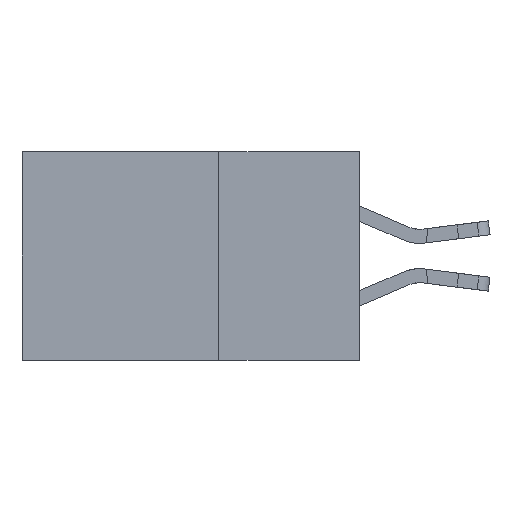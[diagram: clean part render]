
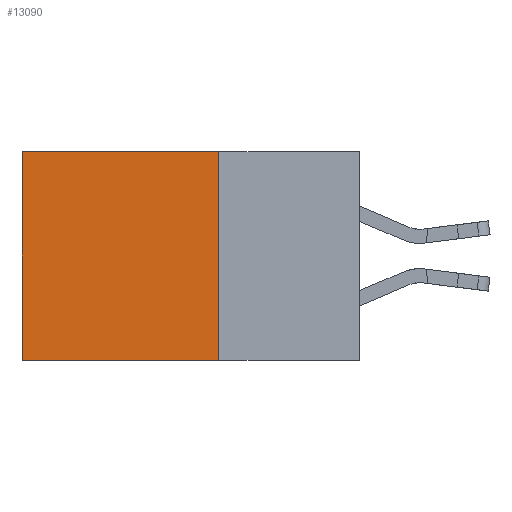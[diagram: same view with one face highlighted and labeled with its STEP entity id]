
A CAD part, left-side view. The second image highlights one B-rep face of the part: STEP entity #13090.
In plain terms, the highlighted planar face has unit normal (-1, 0, 0).
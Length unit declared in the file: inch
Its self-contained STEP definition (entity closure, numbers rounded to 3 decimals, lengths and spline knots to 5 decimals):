
#671 = CARTESIAN_POINT ( 'NONE',  ( 0.2875, 0.25, -0.37 ) ) ;
#3125 = DIRECTION ( 'NONE',  ( 0., 0., -1. ) ) ;
#3146 = VECTOR ( 'NONE', #27133, 39.37008 ) ;
#5110 = LINE ( 'NONE', #15081, #3146 ) ;
#6224 = LINE ( 'NONE', #28887, #25252 ) ;
#6437 = CARTESIAN_POINT ( 'NONE',  ( 0.2875, 0.25, 0. ) ) ;
#8980 = VERTEX_POINT ( 'NONE', #14138 ) ;
#8996 = PLANE ( 'NONE',  #17904 ) ;
#9022 = DIRECTION ( 'NONE',  ( 0., 1., 0. ) ) ;
#9914 = CARTESIAN_POINT ( 'NONE',  ( 0.2875, 0.6, 0. ) ) ;
#11239 = DIRECTION ( 'NONE',  ( 0., 0., -1. ) ) ;
#11529 = DIRECTION ( 'NONE',  ( 0., 0., -1. ) ) ;
#13090 = ADVANCED_FACE ( 'NONE', ( #13191 ), #8996, .F. ) ;
#13191 = FACE_OUTER_BOUND ( 'NONE', #18414, .T. ) ;
#14138 = CARTESIAN_POINT ( 'NONE',  ( 0.2875, 0.25, 0. ) ) ;
#14411 = ORIENTED_EDGE ( 'NONE', *, *, #16341, .T. ) ;
#15081 = CARTESIAN_POINT ( 'NONE',  ( 0.2875, 0.25, -0.37 ) ) ;
#16036 = CARTESIAN_POINT ( 'NONE',  ( 0.2875, 0.6, 0. ) ) ;
#16063 = VERTEX_POINT ( 'NONE', #16036 ) ;
#16341 = EDGE_CURVE ( 'NONE', #16063, #16381, #24700, .T. ) ;
#16381 = VERTEX_POINT ( 'NONE', #17940 ) ;
#17106 = EDGE_CURVE ( 'NONE', #8980, #30665, #6224, .T. ) ;
#17653 = ORIENTED_EDGE ( 'NONE', *, *, #24372, .F. ) ;
#17904 = AXIS2_PLACEMENT_3D ( 'NONE', #18173, #27974, #11239 ) ;
#17940 = CARTESIAN_POINT ( 'NONE',  ( 0.2875, 0.6, -0.37 ) ) ;
#18173 = CARTESIAN_POINT ( 'NONE',  ( 0.2875, 0.25, 0. ) ) ;
#18414 = EDGE_LOOP ( 'NONE', ( #14411, #17653, #30428, #19377 ) ) ;
#19377 = ORIENTED_EDGE ( 'NONE', *, *, #21065, .T. ) ;
#20234 = VECTOR ( 'NONE', #9022, 39.37008 ) ;
#21065 = EDGE_CURVE ( 'NONE', #8980, #16063, #31196, .T. ) ;
#24372 = EDGE_CURVE ( 'NONE', #30665, #16381, #5110, .T. ) ;
#24700 = LINE ( 'NONE', #9914, #24720 ) ;
#24720 = VECTOR ( 'NONE', #3125, 39.37008 ) ;
#25252 = VECTOR ( 'NONE', #11529, 39.37008 ) ;
#27133 = DIRECTION ( 'NONE',  ( 0., 1., 0. ) ) ;
#27974 = DIRECTION ( 'NONE',  ( 1., 0., 0. ) ) ;
#28887 = CARTESIAN_POINT ( 'NONE',  ( 0.2875, 0.25, 0. ) ) ;
#30428 = ORIENTED_EDGE ( 'NONE', *, *, #17106, .F. ) ;
#30665 = VERTEX_POINT ( 'NONE', #671 ) ;
#31196 = LINE ( 'NONE', #6437, #20234 ) ;
